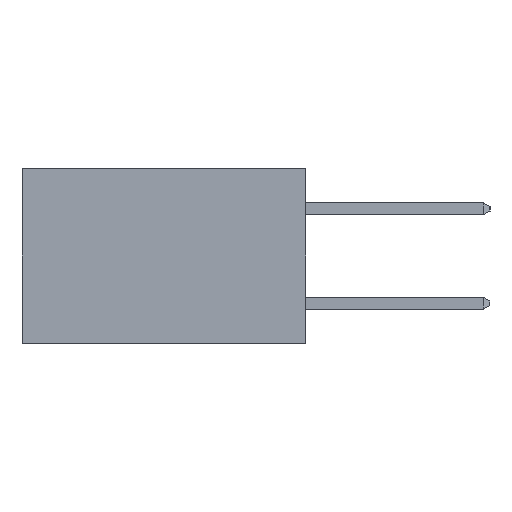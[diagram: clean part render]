
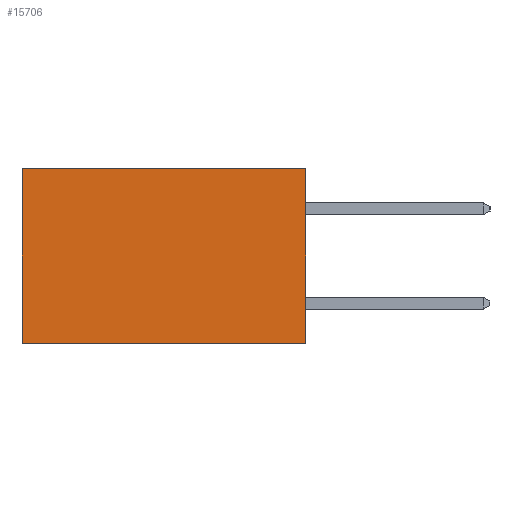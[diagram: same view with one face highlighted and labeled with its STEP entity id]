
A CAD part, left-side view. The second image highlights one B-rep face of the part: STEP entity #15706.
In plain terms, the highlighted planar face has unit normal (-1, 0, 0).
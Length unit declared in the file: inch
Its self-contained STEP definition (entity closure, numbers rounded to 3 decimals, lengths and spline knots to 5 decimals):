
#178 = CARTESIAN_POINT ( 'NONE',  ( 0.298, 0.6, 0. ) ) ;
#311 = EDGE_CURVE ( 'NONE', #11027, #10737, #10920, .T. ) ;
#1127 = LINE ( 'NONE', #9666, #5044 ) ;
#1202 = CARTESIAN_POINT ( 'NONE',  ( 0.298, 0.6, 0. ) ) ;
#2464 = DIRECTION ( 'NONE',  ( 0., 1., 0. ) ) ;
#3224 = ORIENTED_EDGE ( 'NONE', *, *, #5927, .T. ) ;
#3302 = PLANE ( 'NONE',  #13069 ) ;
#4623 = CARTESIAN_POINT ( 'NONE',  ( 0.298, 0., -0.37 ) ) ;
#5044 = VECTOR ( 'NONE', #14237, 39.37008 ) ;
#5340 = CARTESIAN_POINT ( 'NONE',  ( 0.298, 0., -0.37 ) ) ;
#5363 = VERTEX_POINT ( 'NONE', #11998 ) ;
#5369 = LINE ( 'NONE', #1202, #13567 ) ;
#5927 = EDGE_CURVE ( 'NONE', #5363, #18236, #7429, .T. ) ;
#5999 = CARTESIAN_POINT ( 'NONE',  ( 0.298, 0., 0. ) ) ;
#6448 = EDGE_CURVE ( 'NONE', #18236, #10737, #5369, .T. ) ;
#6606 = CARTESIAN_POINT ( 'NONE',  ( 0.298, 0., 0. ) ) ;
#7429 = LINE ( 'NONE', #5999, #14613 ) ;
#8125 = DIRECTION ( 'NONE',  ( 0., 0., -1. ) ) ;
#9319 = EDGE_LOOP ( 'NONE', ( #12224, #10804, #18768, #3224 ) ) ;
#9666 = CARTESIAN_POINT ( 'NONE',  ( 0.298, 0., 0. ) ) ;
#9969 = EDGE_CURVE ( 'NONE', #5363, #11027, #1127, .T. ) ;
#10737 = VERTEX_POINT ( 'NONE', #15588 ) ;
#10804 = ORIENTED_EDGE ( 'NONE', *, *, #311, .F. ) ;
#10920 = LINE ( 'NONE', #4623, #13083 ) ;
#11027 = VERTEX_POINT ( 'NONE', #5340 ) ;
#11998 = CARTESIAN_POINT ( 'NONE',  ( 0.298, 0., 0. ) ) ;
#12169 = DIRECTION ( 'NONE',  ( 0., 1., 0. ) ) ;
#12224 = ORIENTED_EDGE ( 'NONE', *, *, #6448, .T. ) ;
#12284 = DIRECTION ( 'NONE',  ( 0., 0., -1. ) ) ;
#13069 = AXIS2_PLACEMENT_3D ( 'NONE', #6606, #17178, #8125 ) ;
#13083 = VECTOR ( 'NONE', #2464, 39.37008 ) ;
#13567 = VECTOR ( 'NONE', #12284, 39.37008 ) ;
#14237 = DIRECTION ( 'NONE',  ( 0., 0., -1. ) ) ;
#14613 = VECTOR ( 'NONE', #12169, 39.37008 ) ;
#15588 = CARTESIAN_POINT ( 'NONE',  ( 0.298, 0.6, -0.37 ) ) ;
#15706 = ADVANCED_FACE ( 'NONE', ( #16964 ), #3302, .F. ) ;
#16964 = FACE_OUTER_BOUND ( 'NONE', #9319, .T. ) ;
#17178 = DIRECTION ( 'NONE',  ( 1., 0., 0. ) ) ;
#18236 = VERTEX_POINT ( 'NONE', #178 ) ;
#18768 = ORIENTED_EDGE ( 'NONE', *, *, #9969, .F. ) ;
